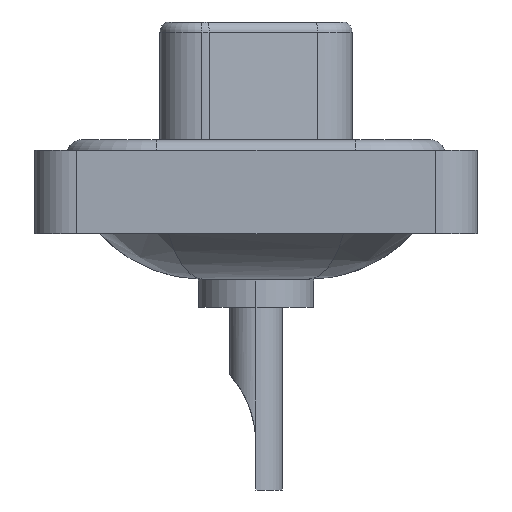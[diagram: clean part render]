
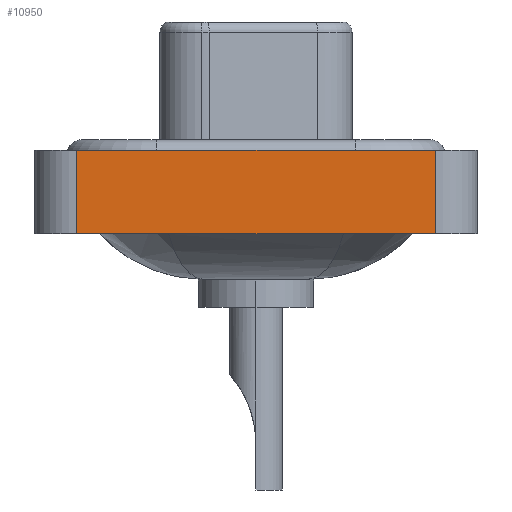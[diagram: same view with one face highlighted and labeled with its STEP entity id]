
A CAD part, left-side view. The second image highlights one B-rep face of the part: STEP entity #10950.
In plain terms, the highlighted planar face has unit normal (-1, 0, 0).
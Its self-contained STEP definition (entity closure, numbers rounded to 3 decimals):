
#377 = CARTESIAN_POINT ( 'NONE',  ( -7.25, -8.55, -3.6 ) ) ;
#378 = LINE ( 'NONE', #6285, #16338 ) ;
#464 = PLANE ( 'NONE',  #18058 ) ;
#705 = CARTESIAN_POINT ( 'NONE',  ( -7.25, 8.55, 0.4 ) ) ;
#761 = EDGE_CURVE ( 'NONE', #3602, #12646, #2739, .T. ) ;
#1282 = EDGE_CURVE ( 'NONE', #16362, #12646, #378, .T. ) ;
#1862 = DIRECTION ( 'NONE',  ( -1., 0., 0. ) ) ;
#2028 = DIRECTION ( 'NONE',  ( 0., 0., 1. ) ) ;
#2209 = DIRECTION ( 'NONE',  ( 0., 0., 1. ) ) ;
#2739 = LINE ( 'NONE', #8187, #14294 ) ;
#3127 = EDGE_CURVE ( 'NONE', #7721, #16362, #8658, .T. ) ;
#3602 = VERTEX_POINT ( 'NONE', #705 ) ;
#3643 = ORIENTED_EDGE ( 'NONE', *, *, #17588, .F. ) ;
#4123 = CARTESIAN_POINT ( 'NONE',  ( -7.25, -8.55, -3.6 ) ) ;
#5002 = ORIENTED_EDGE ( 'NONE', *, *, #761, .F. ) ;
#5245 = ORIENTED_EDGE ( 'NONE', *, *, #3127, .T. ) ;
#6285 = CARTESIAN_POINT ( 'NONE',  ( -7.25, -8.55, -3.6 ) ) ;
#7646 = CARTESIAN_POINT ( 'NONE',  ( -7.25, 8.55, -3.6 ) ) ;
#7721 = VERTEX_POINT ( 'NONE', #9787 ) ;
#8187 = CARTESIAN_POINT ( 'NONE',  ( -7.25, -8.55, 0.4 ) ) ;
#8445 = DIRECTION ( 'NONE',  ( 0., -1., 0. ) ) ;
#8658 = LINE ( 'NONE', #10202, #13638 ) ;
#9787 = CARTESIAN_POINT ( 'NONE',  ( -7.25, 8.55, -3.6 ) ) ;
#10202 = CARTESIAN_POINT ( 'NONE',  ( -7.25, -8.55, -3.6 ) ) ;
#10950 = ADVANCED_FACE ( 'NONE', ( #13137 ), #464, .T. ) ;
#11958 = DIRECTION ( 'NONE',  ( 0., 0., 1. ) ) ;
#12305 = ORIENTED_EDGE ( 'NONE', *, *, #1282, .T. ) ;
#12646 = VERTEX_POINT ( 'NONE', #15788 ) ;
#13137 = FACE_OUTER_BOUND ( 'NONE', #14655, .T. ) ;
#13638 = VECTOR ( 'NONE', #14410, 1000. ) ;
#14294 = VECTOR ( 'NONE', #8445, 1000. ) ;
#14410 = DIRECTION ( 'NONE',  ( 0., -1., 0. ) ) ;
#14592 = LINE ( 'NONE', #7646, #14749 ) ;
#14655 = EDGE_LOOP ( 'NONE', ( #12305, #5002, #3643, #5245 ) ) ;
#14749 = VECTOR ( 'NONE', #2028, 1000. ) ;
#15788 = CARTESIAN_POINT ( 'NONE',  ( -7.25, -8.55, 0.4 ) ) ;
#16338 = VECTOR ( 'NONE', #2209, 1000. ) ;
#16362 = VERTEX_POINT ( 'NONE', #4123 ) ;
#17588 = EDGE_CURVE ( 'NONE', #7721, #3602, #14592, .T. ) ;
#18058 = AXIS2_PLACEMENT_3D ( 'NONE', #377, #1862, #11958 ) ;
